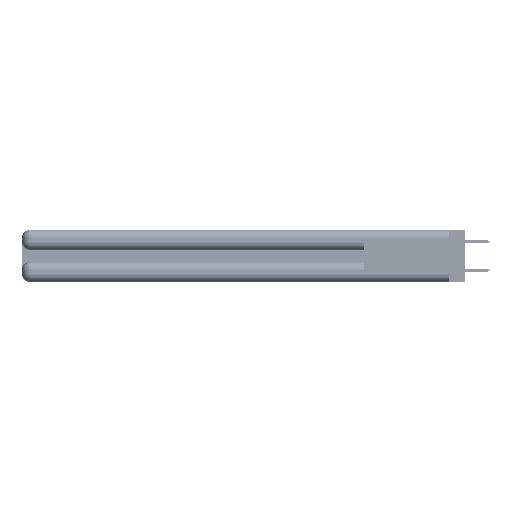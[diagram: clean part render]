
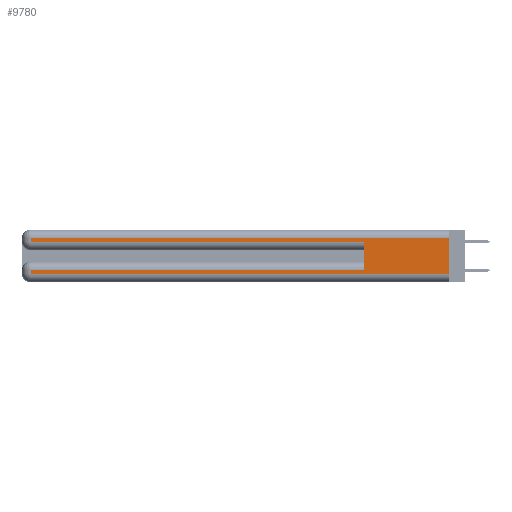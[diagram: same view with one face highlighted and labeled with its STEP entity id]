
A CAD part, left-side view. The second image highlights one B-rep face of the part: STEP entity #9780.
In plain terms, the highlighted planar face has unit normal (-1, 0, 0).
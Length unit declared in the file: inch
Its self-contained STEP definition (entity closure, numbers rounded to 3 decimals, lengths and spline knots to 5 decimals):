
#383 = CARTESIAN_POINT ( 'NONE',  ( 0., 2.94, 0.085 ) ) ;
#1045 = CARTESIAN_POINT ( 'NONE',  ( 0., 2.94, 0.37 ) ) ;
#2442 = CARTESIAN_POINT ( 'NONE',  ( 0., 0., 0.06 ) ) ;
#2473 = ORIENTED_EDGE ( 'NONE', *, *, #47117, .T. ) ;
#4180 = LINE ( 'NONE', #2442, #37351 ) ;
#4980 = ORIENTED_EDGE ( 'NONE', *, *, #30836, .T. ) ;
#5407 = DIRECTION ( 'NONE',  ( 0., 0., -1. ) ) ;
#6479 = CARTESIAN_POINT ( 'NONE',  ( 0., 0.6, 0.145 ) ) ;
#6733 = VERTEX_POINT ( 'NONE', #383 ) ;
#6796 = LINE ( 'NONE', #47905, #55430 ) ;
#7714 = ORIENTED_EDGE ( 'NONE', *, *, #11650, .F. ) ;
#7939 = CARTESIAN_POINT ( 'NONE',  ( 0., 2.94, 0.37 ) ) ;
#7975 = FACE_OUTER_BOUND ( 'NONE', #43680, .T. ) ;
#7980 = EDGE_CURVE ( 'NONE', #6733, #47430, #54121, .T. ) ;
#9248 = LINE ( 'NONE', #14756, #41036 ) ;
#9579 = CARTESIAN_POINT ( 'NONE',  ( 0., 0.6, 0.285 ) ) ;
#9679 = CARTESIAN_POINT ( 'NONE',  ( 0., 2.94, 0.31 ) ) ;
#9780 = ADVANCED_FACE ( 'NONE', ( #7975 ), #15365, .F. ) ;
#10222 = EDGE_CURVE ( 'NONE', #44465, #44479, #9248, .T. ) ;
#10797 = VERTEX_POINT ( 'NONE', #9579 ) ;
#10852 = DIRECTION ( 'NONE',  ( 0., 0., 1. ) ) ;
#11650 = EDGE_CURVE ( 'NONE', #53864, #10797, #32125, .T. ) ;
#13380 = DIRECTION ( 'NONE',  ( 0., 1., 0. ) ) ;
#14320 = CARTESIAN_POINT ( 'NONE',  ( 0., 0., 0.085 ) ) ;
#14515 = ORIENTED_EDGE ( 'NONE', *, *, #43790, .T. ) ;
#14756 = CARTESIAN_POINT ( 'NONE',  ( 0., 0., 0.37 ) ) ;
#15365 = PLANE ( 'NONE',  #17083 ) ;
#15556 = CARTESIAN_POINT ( 'NONE',  ( 0., 0., 0.37 ) ) ;
#17083 = AXIS2_PLACEMENT_3D ( 'NONE', #15556, #45741, #19908 ) ;
#17112 = CARTESIAN_POINT ( 'NONE',  ( 0., 2.94, 0.285 ) ) ;
#18681 = DIRECTION ( 'NONE',  ( 0., 1., 0. ) ) ;
#19908 = DIRECTION ( 'NONE',  ( 0., 0., -1. ) ) ;
#21727 = VECTOR ( 'NONE', #18681, 39.37008 ) ;
#26851 = EDGE_CURVE ( 'NONE', #27425, #32375, #51906, .T. ) ;
#26997 = CARTESIAN_POINT ( 'NONE',  ( 0., 0., 0.285 ) ) ;
#27425 = VERTEX_POINT ( 'NONE', #9679 ) ;
#29844 = VECTOR ( 'NONE', #5407, 39.37008 ) ;
#30836 = EDGE_CURVE ( 'NONE', #32375, #10797, #53693, .T. ) ;
#32125 = LINE ( 'NONE', #6479, #39518 ) ;
#32375 = VERTEX_POINT ( 'NONE', #17112 ) ;
#36933 = CARTESIAN_POINT ( 'NONE',  ( 0., 2.94, 0.06 ) ) ;
#36950 = EDGE_CURVE ( 'NONE', #53864, #6733, #55965, .T. ) ;
#37052 = DIRECTION ( 'NONE',  ( 0., -1., 0. ) ) ;
#37351 = VECTOR ( 'NONE', #37052, 39.37008 ) ;
#37543 = CARTESIAN_POINT ( 'NONE',  ( 0., 0., 0.06 ) ) ;
#38325 = ORIENTED_EDGE ( 'NONE', *, *, #26851, .T. ) ;
#39518 = VECTOR ( 'NONE', #10852, 39.37008 ) ;
#40440 = VECTOR ( 'NONE', #42683, 39.37008 ) ;
#41036 = VECTOR ( 'NONE', #53619, 39.37008 ) ;
#41548 = CARTESIAN_POINT ( 'NONE',  ( 0., 0.6, 0.085 ) ) ;
#42162 = ORIENTED_EDGE ( 'NONE', *, *, #36950, .T. ) ;
#42683 = DIRECTION ( 'NONE',  ( 0., 0., -1. ) ) ;
#43036 = ORIENTED_EDGE ( 'NONE', *, *, #10222, .F. ) ;
#43680 = EDGE_LOOP ( 'NONE', ( #43036, #2473, #38325, #4980, #7714, #42162, #54987, #14515 ) ) ;
#43790 = EDGE_CURVE ( 'NONE', #47430, #44479, #4180, .T. ) ;
#44465 = VERTEX_POINT ( 'NONE', #46028 ) ;
#44479 = VERTEX_POINT ( 'NONE', #37543 ) ;
#45741 = DIRECTION ( 'NONE',  ( 1., 0., 0. ) ) ;
#46028 = CARTESIAN_POINT ( 'NONE',  ( 0., 0., 0.31 ) ) ;
#47117 = EDGE_CURVE ( 'NONE', #44465, #27425, #6796, .T. ) ;
#47430 = VERTEX_POINT ( 'NONE', #36933 ) ;
#47905 = CARTESIAN_POINT ( 'NONE',  ( 0., 0., 0.31 ) ) ;
#48513 = DIRECTION ( 'NONE',  ( 0., -1., 0. ) ) ;
#51906 = LINE ( 'NONE', #7939, #40440 ) ;
#52326 = VECTOR ( 'NONE', #48513, 39.37008 ) ;
#53619 = DIRECTION ( 'NONE',  ( 0., 0., -1. ) ) ;
#53693 = LINE ( 'NONE', #26997, #52326 ) ;
#53864 = VERTEX_POINT ( 'NONE', #41548 ) ;
#54121 = LINE ( 'NONE', #1045, #29844 ) ;
#54987 = ORIENTED_EDGE ( 'NONE', *, *, #7980, .T. ) ;
#55430 = VECTOR ( 'NONE', #13380, 39.37008 ) ;
#55965 = LINE ( 'NONE', #14320, #21727 ) ;
